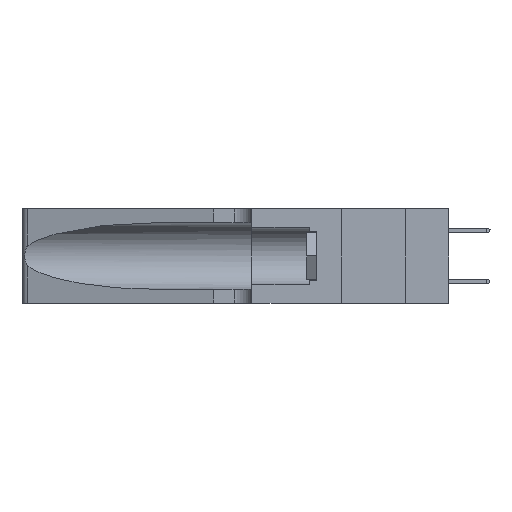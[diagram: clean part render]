
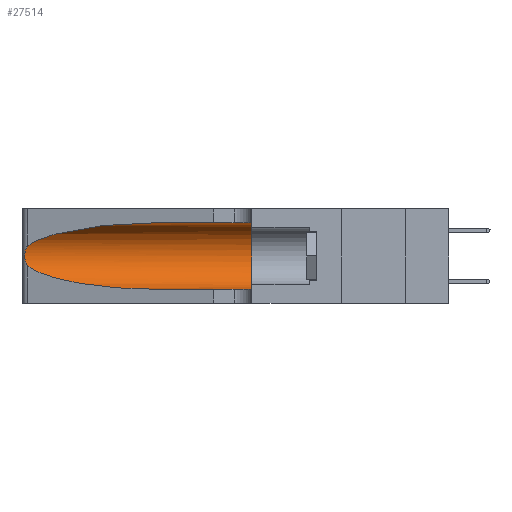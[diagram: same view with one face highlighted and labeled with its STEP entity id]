
A CAD part, left-side view. The second image highlights one B-rep face of the part: STEP entity #27514.
In plain terms, the highlighted cylindrical face has radius 3.308 mm (diameter 6.617 mm), a partial arc.
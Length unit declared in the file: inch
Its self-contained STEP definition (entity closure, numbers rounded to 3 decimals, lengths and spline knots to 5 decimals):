
#1093 = LINE ( 'NONE', #41203, #29954 ) ;
#1216 = EDGE_CURVE ( 'NONE', #13038, #11970, #1093, .T. ) ;
#2247 = EDGE_CURVE ( 'NONE', #13038, #43090, #23666, .T. ) ;
#2870 = CARTESIAN_POINT ( 'NONE',  ( 0.25555, 1.22993, 0.14849 ) ) ;
#5089 = VERTEX_POINT ( 'NONE', #40399 ) ;
#10312 = CARTESIAN_POINT ( 'NONE',  ( 0.25787, 1.23484, 0.2124 ) ) ;
#11076 = EDGE_CURVE ( 'NONE', #43090, #38255, #46081, .T. ) ;
#11970 = VERTEX_POINT ( 'NONE', #42075 ) ;
#13038 = VERTEX_POINT ( 'NONE', #47880 ) ;
#13577 = DIRECTION ( 'NONE',  ( 0., 1., 0. ) ) ;
#13922 = CARTESIAN_POINT ( 'NONE',  ( 0.1305, 0.72297, 0.05475 ) ) ;
#14124 = CARTESIAN_POINT ( 'NONE',  ( 0.26018, 1.23835, 0.19895 ) ) ;
#14325 = ORIENTED_EDGE ( 'NONE', *, *, #1216, .F. ) ;
#15630 = CARTESIAN_POINT ( 'NONE',  ( 0.1305, 1.61858, 0.185 ) ) ;
#17203 = CARTESIAN_POINT ( 'NONE',  ( 0.18966, 0.96281, 0.31525 ) ) ;
#17897 = CARTESIAN_POINT ( 'NONE',  ( 0.26075, 1.23896, 0.178 ) ) ;
#19002 = ORIENTED_EDGE ( 'NONE', *, *, #23546, .F. ) ;
#19058 = ORIENTED_EDGE ( 'NONE', *, *, #27862, .T. ) ;
#19142 = AXIS2_PLACEMENT_3D ( 'NONE', #15630, #41694, #23091 ) ;
#21016 = CARTESIAN_POINT ( 'NONE',  ( 0.25487, 1.22718, 0.22369 ) ) ;
#21218 = ORIENTED_EDGE ( 'NONE', *, *, #2247, .T. ) ;
#21738 = CARTESIAN_POINT ( 'NONE',  ( 0.25856, 1.23593, 0.16098 ) ) ;
#22082 = AXIS2_PLACEMENT_3D ( 'NONE', #35963, #13577, #39668 ) ;
#22540 = CARTESIAN_POINT ( 'NONE',  ( 0.25487, 1.22718, 0.14631 ) ) ;
#22572 = ORIENTED_EDGE ( 'NONE', *, *, #11076, .T. ) ;
#23091 = DIRECTION ( 'NONE',  ( 0., 0., -1. ) ) ;
#23546 = EDGE_CURVE ( 'NONE', #11970, #5089, #26728, .T. ) ;
#23666 =( BOUNDED_CURVE ( )  B_SPLINE_CURVE ( 3, ( #43205, #17203, #35801, #21016 ),
 .UNSPECIFIED., .F., .F. ) 
 B_SPLINE_CURVE_WITH_KNOTS ( ( 4, 4 ),
 ( 1.5708, 2.84003 ),
 .UNSPECIFIED. ) 
 CURVE ( )  GEOMETRIC_REPRESENTATION_ITEM ( )  RATIONAL_B_SPLINE_CURVE ( ( 1., 0.87, 0.87, 1. ) ) 
 REPRESENTATION_ITEM ( '' )  );
#24430 = EDGE_LOOP ( 'NONE', ( #21218, #22572, #45772, #19058, #19002, #14325 ) ) ;
#25102 = CARTESIAN_POINT ( 'NONE',  ( 0.25487, 1.22718, 0.14631 ) ) ;
#25169 = FACE_OUTER_BOUND ( 'NONE', #24430, .T. ) ;
#25306 = CARTESIAN_POINT ( 'NONE',  ( 0.25487, 1.22718, 0.22369 ) ) ;
#25461 = CARTESIAN_POINT ( 'NONE',  ( 0.25639, 1.23186, 0.15144 ) ) ;
#25753 =( BOUNDED_CURVE ( )  B_SPLINE_CURVE ( 3, ( #25102, #47223, #36292, #13922 ),
 .UNSPECIFIED., .F., .F. ) 
 B_SPLINE_CURVE_WITH_KNOTS ( ( 4, 4 ),
 ( 3.44316, 4.71239 ),
 .UNSPECIFIED. ) 
 CURVE ( )  GEOMETRIC_REPRESENTATION_ITEM ( )  RATIONAL_B_SPLINE_CURVE ( ( 1., 0.87, 0.87, 1. ) ) 
 REPRESENTATION_ITEM ( '' )  );
#26494 = EDGE_CURVE ( 'NONE', #38255, #44880, #25753, .T. ) ;
#26728 = CIRCLE ( 'NONE', #22082, 0.13025 ) ;
#27514 = ADVANCED_FACE ( 'NONE', ( #25169 ), #43688, .F. ) ;
#27862 = EDGE_CURVE ( 'NONE', #44880, #5089, #29790, .T. ) ;
#29187 = CARTESIAN_POINT ( 'NONE',  ( 0.25487, 1.22718, 0.14631 ) ) ;
#29790 = LINE ( 'NONE', #36182, #48201 ) ;
#29954 = VECTOR ( 'NONE', #41365, 39.37008 ) ;
#32279 = CARTESIAN_POINT ( 'NONE',  ( 0.25487, 1.22718, 0.22369 ) ) ;
#32777 = CARTESIAN_POINT ( 'NONE',  ( 0.25639, 1.23184, 0.21858 ) ) ;
#33560 = CARTESIAN_POINT ( 'NONE',  ( 0.1305, 0.72297, 0.05475 ) ) ;
#35801 = CARTESIAN_POINT ( 'NONE',  ( 0.2373, 1.15595, 0.28018 ) ) ;
#35963 = CARTESIAN_POINT ( 'NONE',  ( 0.1305, 0.35, 0.185 ) ) ;
#36182 = CARTESIAN_POINT ( 'NONE',  ( 0.1305, 1.61858, 0.05475 ) ) ;
#36292 = CARTESIAN_POINT ( 'NONE',  ( 0.18966, 0.96281, 0.05475 ) ) ;
#36493 = CARTESIAN_POINT ( 'NONE',  ( 0.25854, 1.2359, 0.20912 ) ) ;
#38255 = VERTEX_POINT ( 'NONE', #22540 ) ;
#39668 = DIRECTION ( 'NONE',  ( 0., 0., 1. ) ) ;
#39884 = DIRECTION ( 'NONE',  ( 0., -1., 0. ) ) ;
#40192 = CARTESIAN_POINT ( 'NONE',  ( 0.26075, 1.23896, 0.19203 ) ) ;
#40399 = CARTESIAN_POINT ( 'NONE',  ( 0.1305, 0.35, 0.05475 ) ) ;
#41203 = CARTESIAN_POINT ( 'NONE',  ( 0.1305, 1.61858, 0.31525 ) ) ;
#41365 = DIRECTION ( 'NONE',  ( 0., -1., 0. ) ) ;
#41694 = DIRECTION ( 'NONE',  ( 0., -1., 0. ) ) ;
#42075 = CARTESIAN_POINT ( 'NONE',  ( 0.1305, 0.35, 0.31525 ) ) ;
#43090 = VERTEX_POINT ( 'NONE', #32279 ) ;
#43205 = CARTESIAN_POINT ( 'NONE',  ( 0.1305, 0.72297, 0.31525 ) ) ;
#43688 = CYLINDRICAL_SURFACE ( 'NONE', #19142, 0.13025 ) ;
#43906 = CARTESIAN_POINT ( 'NONE',  ( 0.26017, 1.23833, 0.17102 ) ) ;
#44880 = VERTEX_POINT ( 'NONE', #33560 ) ;
#45772 = ORIENTED_EDGE ( 'NONE', *, *, #26494, .T. ) ;
#46081 = B_SPLINE_CURVE_WITH_KNOTS ( 'NONE', 3,
 ( #25306, #47411, #32777, #10312, #36493, #14124, #40192, #17897, #43906, #21738, #47564, #25461, #2870, #29187 ),
 .UNSPECIFIED., .F., .F.,
 ( 4, 2, 2, 2, 2, 2, 4 ),
 ( 0., 0.00027, 0.00053, 0.00107, 0.0016, 0.00187, 0.00214 ),
 .UNSPECIFIED. ) ;
#47223 = CARTESIAN_POINT ( 'NONE',  ( 0.2373, 1.15595, 0.08982 ) ) ;
#47411 = CARTESIAN_POINT ( 'NONE',  ( 0.25555, 1.22994, 0.2215 ) ) ;
#47564 = CARTESIAN_POINT ( 'NONE',  ( 0.25789, 1.23486, 0.15765 ) ) ;
#47880 = CARTESIAN_POINT ( 'NONE',  ( 0.1305, 0.72297, 0.31525 ) ) ;
#48201 = VECTOR ( 'NONE', #39884, 39.37008 ) ;
